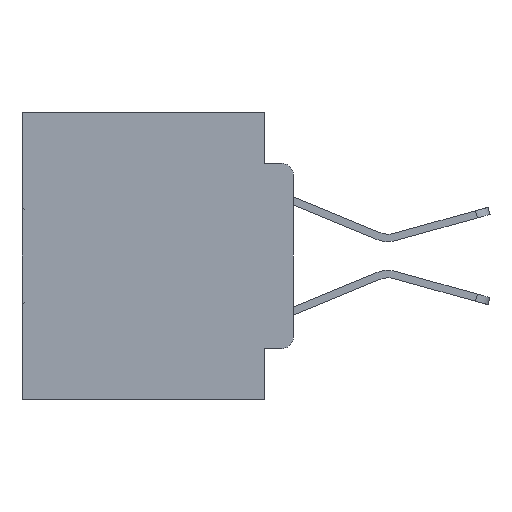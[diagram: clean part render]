
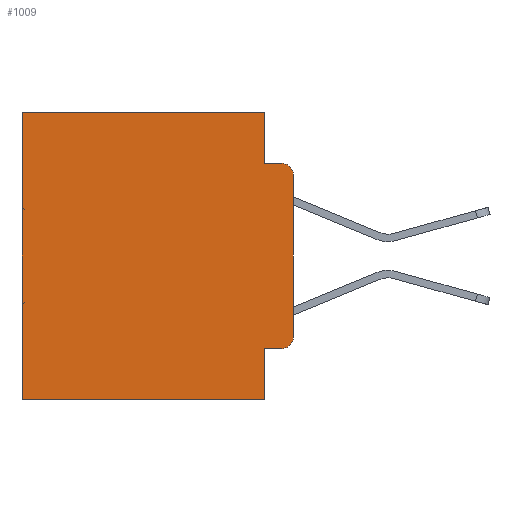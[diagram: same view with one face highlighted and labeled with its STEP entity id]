
A CAD part, left-side view. The second image highlights one B-rep face of the part: STEP entity #1009.
In plain terms, the highlighted planar face has unit normal (-1, 0, 0).
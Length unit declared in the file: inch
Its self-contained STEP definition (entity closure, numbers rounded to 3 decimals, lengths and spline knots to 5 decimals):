
#372 = DIRECTION ( 'NONE',  ( 0., -1., 0. ) ) ;
#752 = CARTESIAN_POINT ( 'NONE',  ( 0.298, 0.473, -0.5 ) ) ;
#1009 = ADVANCED_FACE ( 'NONE', ( #25092 ), #16788, .F. ) ;
#1348 = VERTEX_POINT ( 'NONE', #14219 ) ;
#1943 = CARTESIAN_POINT ( 'NONE',  ( 0.298, 0.051, 0. ) ) ;
#2118 = EDGE_CURVE ( 'NONE', #17830, #10243, #5091, .T. ) ;
#3618 = VECTOR ( 'NONE', #15910, 39.37008 ) ;
#3626 = ORIENTED_EDGE ( 'NONE', *, *, #31515, .T. ) ;
#4053 = ORIENTED_EDGE ( 'NONE', *, *, #29801, .F. ) ;
#5091 = CIRCLE ( 'NONE', #8967, 0.02 ) ;
#5180 = VECTOR ( 'NONE', #372, 39.37008 ) ;
#5428 = VERTEX_POINT ( 'NONE', #12645 ) ;
#5727 = ORIENTED_EDGE ( 'NONE', *, *, #28379, .F. ) ;
#8496 = CIRCLE ( 'NONE', #16753, 0.02 ) ;
#8967 = AXIS2_PLACEMENT_3D ( 'NONE', #32242, #32163, #20307 ) ;
#9748 = VECTOR ( 'NONE', #27833, 39.37008 ) ;
#9793 = VERTEX_POINT ( 'NONE', #26517 ) ;
#10023 = CARTESIAN_POINT ( 'NONE',  ( 0.298, 0.02, -0.3915 ) ) ;
#10243 = VERTEX_POINT ( 'NONE', #23349 ) ;
#10263 = ORIENTED_EDGE ( 'NONE', *, *, #30562, .F. ) ;
#10624 = CARTESIAN_POINT ( 'NONE',  ( 0.298, 0., 0. ) ) ;
#10664 = LINE ( 'NONE', #18383, #3618 ) ;
#10675 = LINE ( 'NONE', #12223, #11480 ) ;
#11005 = CARTESIAN_POINT ( 'NONE',  ( 0.298, 0.051, -0.5 ) ) ;
#11480 = VECTOR ( 'NONE', #14813, 39.37008 ) ;
#11949 = EDGE_CURVE ( 'NONE', #14732, #17329, #16564, .T. ) ;
#12198 = CARTESIAN_POINT ( 'NONE',  ( 0.298, 0.051, -0.0885 ) ) ;
#12223 = CARTESIAN_POINT ( 'NONE',  ( 0.298, 0.473, 0. ) ) ;
#12624 = DIRECTION ( 'NONE',  ( 0., 0., -1. ) ) ;
#12645 = CARTESIAN_POINT ( 'NONE',  ( 0.298, 0.473, 0. ) ) ;
#13988 = LINE ( 'NONE', #28261, #26782 ) ;
#14219 = CARTESIAN_POINT ( 'NONE',  ( 0.298, 0.051, -0.4115 ) ) ;
#14732 = VERTEX_POINT ( 'NONE', #24789 ) ;
#14772 = CARTESIAN_POINT ( 'NONE',  ( 0.298, 0.051, -0.0885 ) ) ;
#14813 = DIRECTION ( 'NONE',  ( 0., 0., -1. ) ) ;
#14988 = VERTEX_POINT ( 'NONE', #11005 ) ;
#15910 = DIRECTION ( 'NONE',  ( 0., 0., -1. ) ) ;
#16280 = ORIENTED_EDGE ( 'NONE', *, *, #18779, .T. ) ;
#16470 = VERTEX_POINT ( 'NONE', #29171 ) ;
#16564 = LINE ( 'NONE', #1943, #9748 ) ;
#16701 = ORIENTED_EDGE ( 'NONE', *, *, #22433, .T. ) ;
#16753 = AXIS2_PLACEMENT_3D ( 'NONE', #10023, #27924, #12624 ) ;
#16788 = PLANE ( 'NONE',  #17775 ) ;
#16850 = VECTOR ( 'NONE', #22464, 39.37008 ) ;
#17329 = VERTEX_POINT ( 'NONE', #12198 ) ;
#17330 = LINE ( 'NONE', #14772, #23308 ) ;
#17516 = DIRECTION ( 'NONE',  ( 0., 1., 0. ) ) ;
#17775 = AXIS2_PLACEMENT_3D ( 'NONE', #10624, #24516, #25422 ) ;
#17830 = VERTEX_POINT ( 'NONE', #27136 ) ;
#18009 = DIRECTION ( 'NONE',  ( 0., 0., -1. ) ) ;
#18168 = LINE ( 'NONE', #31293, #5180 ) ;
#18383 = CARTESIAN_POINT ( 'NONE',  ( 0.298, 0., 0. ) ) ;
#18779 = EDGE_CURVE ( 'NONE', #5428, #27980, #10675, .T. ) ;
#19930 = CARTESIAN_POINT ( 'NONE',  ( 0.298, 0., 0. ) ) ;
#20307 = DIRECTION ( 'NONE',  ( 0., 0., -1. ) ) ;
#22268 = ORIENTED_EDGE ( 'NONE', *, *, #27137, .F. ) ;
#22433 = EDGE_CURVE ( 'NONE', #9793, #16470, #8496, .T. ) ;
#22464 = DIRECTION ( 'NONE',  ( 0., 1., 0. ) ) ;
#22512 = CARTESIAN_POINT ( 'NONE',  ( 0.298, 0., -0.5 ) ) ;
#23308 = VECTOR ( 'NONE', #29990, 39.37008 ) ;
#23349 = CARTESIAN_POINT ( 'NONE',  ( 0.298, 0.02, -0.0885 ) ) ;
#24516 = DIRECTION ( 'NONE',  ( 1., 0., 0. ) ) ;
#24686 = ORIENTED_EDGE ( 'NONE', *, *, #28209, .T. ) ;
#24789 = CARTESIAN_POINT ( 'NONE',  ( 0.298, 0.051, 0. ) ) ;
#25092 = FACE_OUTER_BOUND ( 'NONE', #27999, .T. ) ;
#25422 = DIRECTION ( 'NONE',  ( 0., 0., -1. ) ) ;
#25498 = ORIENTED_EDGE ( 'NONE', *, *, #2118, .T. ) ;
#26517 = CARTESIAN_POINT ( 'NONE',  ( 0.298, 0.02, -0.4115 ) ) ;
#26782 = VECTOR ( 'NONE', #18009, 39.37008 ) ;
#27136 = CARTESIAN_POINT ( 'NONE',  ( 0.298, 0., -0.1085 ) ) ;
#27137 = EDGE_CURVE ( 'NONE', #17329, #10243, #17330, .T. ) ;
#27425 = LINE ( 'NONE', #22512, #33262 ) ;
#27833 = DIRECTION ( 'NONE',  ( 0., 0., -1. ) ) ;
#27924 = DIRECTION ( 'NONE',  ( -1., 0., 0. ) ) ;
#27980 = VERTEX_POINT ( 'NONE', #752 ) ;
#27999 = EDGE_LOOP ( 'NONE', ( #4053, #25498, #22268, #29005, #24686, #16280, #10263, #5727, #3626, #16701 ) ) ;
#28209 = EDGE_CURVE ( 'NONE', #14732, #5428, #30365, .T. ) ;
#28261 = CARTESIAN_POINT ( 'NONE',  ( 0.298, 0.051, 0. ) ) ;
#28379 = EDGE_CURVE ( 'NONE', #1348, #14988, #13988, .T. ) ;
#29005 = ORIENTED_EDGE ( 'NONE', *, *, #11949, .F. ) ;
#29171 = CARTESIAN_POINT ( 'NONE',  ( 0.298, 0., -0.3915 ) ) ;
#29801 = EDGE_CURVE ( 'NONE', #17830, #16470, #10664, .T. ) ;
#29990 = DIRECTION ( 'NONE',  ( 0., -1., 0. ) ) ;
#30365 = LINE ( 'NONE', #19930, #16850 ) ;
#30562 = EDGE_CURVE ( 'NONE', #14988, #27980, #27425, .T. ) ;
#31293 = CARTESIAN_POINT ( 'NONE',  ( 0.298, 0.051, -0.4115 ) ) ;
#31515 = EDGE_CURVE ( 'NONE', #1348, #9793, #18168, .T. ) ;
#32163 = DIRECTION ( 'NONE',  ( -1., 0., 0. ) ) ;
#32242 = CARTESIAN_POINT ( 'NONE',  ( 0.298, 0.02, -0.1085 ) ) ;
#33262 = VECTOR ( 'NONE', #17516, 39.37008 ) ;
